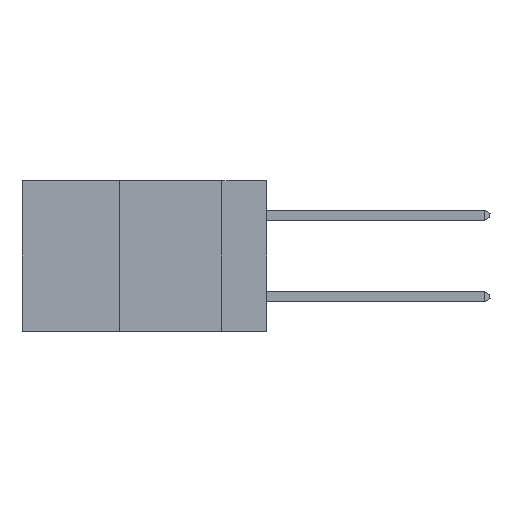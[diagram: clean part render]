
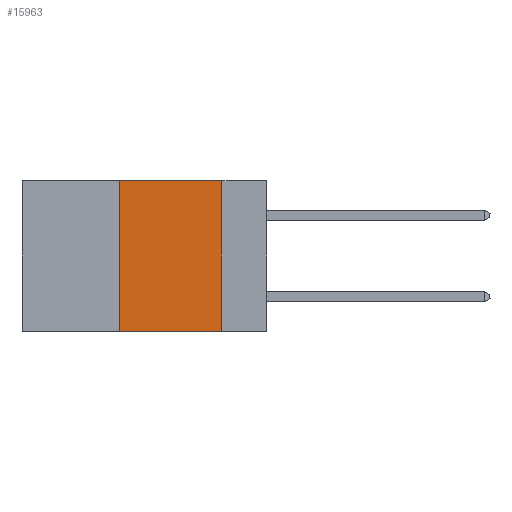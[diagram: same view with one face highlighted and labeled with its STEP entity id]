
A CAD part, left-side view. The second image highlights one B-rep face of the part: STEP entity #15963.
In plain terms, the highlighted planar face has unit normal (-1, 0, 0).
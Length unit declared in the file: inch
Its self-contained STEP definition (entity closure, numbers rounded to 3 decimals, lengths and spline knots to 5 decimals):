
#194 = CARTESIAN_POINT ( 'NONE',  ( 0., 0.36, 0. ) ) ;
#528 = VECTOR ( 'NONE', #22829, 39.37008 ) ;
#1112 = DIRECTION ( 'NONE',  ( 0., -1., 0. ) ) ;
#1128 = LINE ( 'NONE', #21092, #528 ) ;
#1209 = CARTESIAN_POINT ( 'NONE',  ( 0., 0.6, 0. ) ) ;
#2211 = ORIENTED_EDGE ( 'NONE', *, *, #15390, .F. ) ;
#2220 = CARTESIAN_POINT ( 'NONE',  ( 0., 0.36, -0.37 ) ) ;
#2258 = ORIENTED_EDGE ( 'NONE', *, *, #10198, .F. ) ;
#2429 = ORIENTED_EDGE ( 'NONE', *, *, #9855, .F. ) ;
#2482 = ORIENTED_EDGE ( 'NONE', *, *, #13026, .T. ) ;
#3237 = DIRECTION ( 'NONE',  ( 0., -1., 0. ) ) ;
#3369 = DIRECTION ( 'NONE',  ( 1., 0., 0. ) ) ;
#4958 = VERTEX_POINT ( 'NONE', #6889 ) ;
#6726 = CARTESIAN_POINT ( 'NONE',  ( 0., 0.6, -0.37 ) ) ;
#6889 = CARTESIAN_POINT ( 'NONE',  ( 0., 0.11, 0. ) ) ;
#7985 = CARTESIAN_POINT ( 'NONE',  ( 0., 0.36, 0. ) ) ;
#8277 = LINE ( 'NONE', #1209, #13083 ) ;
#9818 = DIRECTION ( 'NONE',  ( 0., 0., 1. ) ) ;
#9855 = EDGE_CURVE ( 'NONE', #14592, #21245, #14492, .T. ) ;
#10198 = EDGE_CURVE ( 'NONE', #21245, #4958, #8277, .T. ) ;
#12265 = VERTEX_POINT ( 'NONE', #20552 ) ;
#13026 = EDGE_CURVE ( 'NONE', #14592, #12265, #19761, .T. ) ;
#13083 = VECTOR ( 'NONE', #3237, 39.37008 ) ;
#14492 = LINE ( 'NONE', #7985, #23092 ) ;
#14592 = VERTEX_POINT ( 'NONE', #2220 ) ;
#15390 = EDGE_CURVE ( 'NONE', #4958, #12265, #1128, .T. ) ;
#15963 = ADVANCED_FACE ( 'NONE', ( #21625 ), #15984, .F. ) ;
#15984 = PLANE ( 'NONE',  #22964 ) ;
#16051 = DIRECTION ( 'NONE',  ( 0., 0., -1. ) ) ;
#19220 = VECTOR ( 'NONE', #1112, 39.37008 ) ;
#19761 = LINE ( 'NONE', #6726, #19220 ) ;
#20552 = CARTESIAN_POINT ( 'NONE',  ( 0., 0.11, -0.37 ) ) ;
#21092 = CARTESIAN_POINT ( 'NONE',  ( 0., 0.11, 0. ) ) ;
#21112 = EDGE_LOOP ( 'NONE', ( #2211, #2258, #2429, #2482 ) ) ;
#21245 = VERTEX_POINT ( 'NONE', #194 ) ;
#21625 = FACE_OUTER_BOUND ( 'NONE', #21112, .T. ) ;
#22829 = DIRECTION ( 'NONE',  ( 0., 0., -1. ) ) ;
#22885 = CARTESIAN_POINT ( 'NONE',  ( 0., 0.6, 0. ) ) ;
#22964 = AXIS2_PLACEMENT_3D ( 'NONE', #22885, #3369, #16051 ) ;
#23092 = VECTOR ( 'NONE', #9818, 39.37008 ) ;
